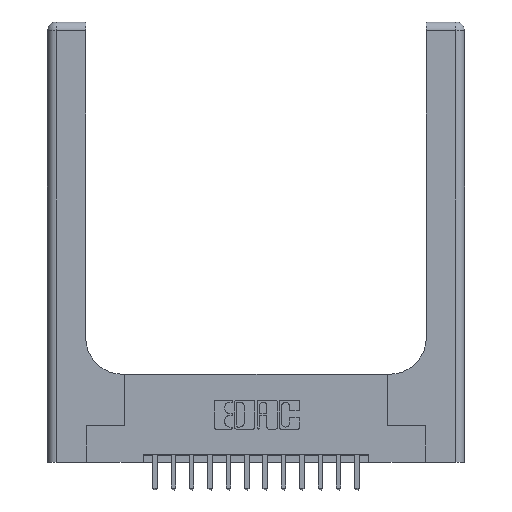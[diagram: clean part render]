
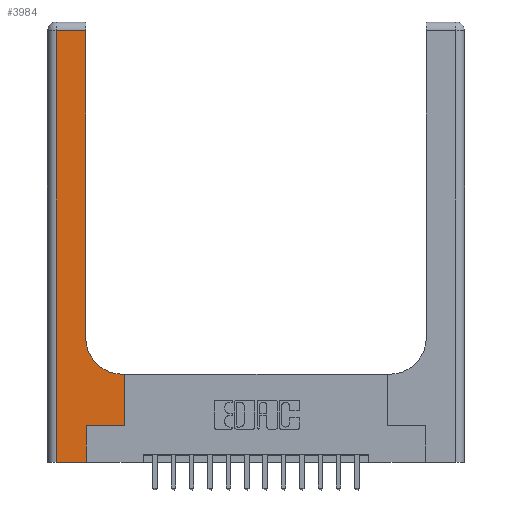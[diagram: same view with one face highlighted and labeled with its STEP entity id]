
A CAD part, top view. The second image highlights one B-rep face of the part: STEP entity #3984.
In plain terms, the highlighted planar face has unit normal (0, 0, 1).
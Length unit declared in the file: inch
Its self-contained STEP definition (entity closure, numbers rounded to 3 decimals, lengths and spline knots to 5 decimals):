
#11 = DIRECTION ( 'NONE',  ( 1., 0., 0. ) ) ;
#186 = LINE ( 'NONE', #16522, #15831 ) ;
#681 = VERTEX_POINT ( 'NONE', #9609 ) ;
#795 = EDGE_LOOP ( 'NONE', ( #807, #1876, #9468, #6690, #6647, #2624, #9070, #843, #6449 ) ) ;
#807 = ORIENTED_EDGE ( 'NONE', *, *, #17196, .T. ) ;
#843 = ORIENTED_EDGE ( 'NONE', *, *, #13848, .T. ) ;
#1026 = DIRECTION ( 'NONE',  ( 0., 1., 0. ) ) ;
#1343 = VERTEX_POINT ( 'NONE', #12396 ) ;
#1766 = DIRECTION ( 'NONE',  ( 0., 1., 0. ) ) ;
#1772 = CARTESIAN_POINT ( 'NONE',  ( 0., 3., 0.37 ) ) ;
#1876 = ORIENTED_EDGE ( 'NONE', *, *, #15842, .T. ) ;
#1943 = LINE ( 'NONE', #8644, #10205 ) ;
#2039 = DIRECTION ( 'NONE',  ( -1., 0., 0. ) ) ;
#2384 = VERTEX_POINT ( 'NONE', #16519 ) ;
#2624 = ORIENTED_EDGE ( 'NONE', *, *, #12705, .T. ) ;
#3038 = CARTESIAN_POINT ( 'NONE',  ( 0., 2.94, 0.37 ) ) ;
#3402 = LINE ( 'NONE', #3038, #15103 ) ;
#3521 = CIRCLE ( 'NONE', #12366, 0.25 ) ;
#3827 = AXIS2_PLACEMENT_3D ( 'NONE', #1772, #5341, #5941 ) ;
#3854 = CARTESIAN_POINT ( 'NONE',  ( 0.26, 3., 0.37 ) ) ;
#3984 = ADVANCED_FACE ( 'NONE', ( #11176 ), #4332, .F. ) ;
#4313 = DIRECTION ( 'NONE',  ( 0., -1., 0. ) ) ;
#4332 = PLANE ( 'NONE',  #3827 ) ;
#4586 = LINE ( 'NONE', #8483, #16909 ) ;
#4690 = CARTESIAN_POINT ( 'NONE',  ( 0.265, 0.25, 0.37 ) ) ;
#5092 = EDGE_CURVE ( 'NONE', #2384, #1343, #3521, .T. ) ;
#5341 = DIRECTION ( 'NONE',  ( 0., 0., -1. ) ) ;
#5524 = VERTEX_POINT ( 'NONE', #4690 ) ;
#5574 = CARTESIAN_POINT ( 'NONE',  ( 0., 0., 0.37 ) ) ;
#5707 = VECTOR ( 'NONE', #7369, 39.37008 ) ;
#5772 = EDGE_CURVE ( 'NONE', #681, #5524, #4586, .T. ) ;
#5941 = DIRECTION ( 'NONE',  ( -1., 0., 0. ) ) ;
#6037 = VERTEX_POINT ( 'NONE', #11807 ) ;
#6064 = EDGE_CURVE ( 'NONE', #12102, #681, #12354, .T. ) ;
#6449 = ORIENTED_EDGE ( 'NONE', *, *, #5092, .T. ) ;
#6647 = ORIENTED_EDGE ( 'NONE', *, *, #5772, .T. ) ;
#6690 = ORIENTED_EDGE ( 'NONE', *, *, #6064, .T. ) ;
#7369 = DIRECTION ( 'NONE',  ( -1., 0., 0. ) ) ;
#7761 = CARTESIAN_POINT ( 'NONE',  ( 0.06, 2.94, 0.37 ) ) ;
#7971 = VERTEX_POINT ( 'NONE', #7761 ) ;
#8050 = VERTEX_POINT ( 'NONE', #14762 ) ;
#8219 = EDGE_CURVE ( 'NONE', #7971, #12102, #186, .T. ) ;
#8483 = CARTESIAN_POINT ( 'NONE',  ( 0.265, 0., 0.37 ) ) ;
#8605 = LINE ( 'NONE', #16819, #5707 ) ;
#8644 = CARTESIAN_POINT ( 'NONE',  ( 0.265, 0.25, 0.37 ) ) ;
#8676 = VECTOR ( 'NONE', #11, 39.37008 ) ;
#9070 = ORIENTED_EDGE ( 'NONE', *, *, #15379, .T. ) ;
#9468 = ORIENTED_EDGE ( 'NONE', *, *, #8219, .T. ) ;
#9609 = CARTESIAN_POINT ( 'NONE',  ( 0.265, 0., 0.37 ) ) ;
#9670 = CARTESIAN_POINT ( 'NONE',  ( 0.26, 2.94, 0.37 ) ) ;
#10205 = VECTOR ( 'NONE', #14080, 39.37008 ) ;
#11176 = FACE_OUTER_BOUND ( 'NONE', #795, .T. ) ;
#11807 = CARTESIAN_POINT ( 'NONE',  ( 0.528, 0.6, 0.37 ) ) ;
#12102 = VERTEX_POINT ( 'NONE', #12962 ) ;
#12287 = VECTOR ( 'NONE', #1026, 39.37008 ) ;
#12354 = LINE ( 'NONE', #5574, #8676 ) ;
#12366 = AXIS2_PLACEMENT_3D ( 'NONE', #17135, #16243, #16161 ) ;
#12396 = CARTESIAN_POINT ( 'NONE',  ( 0.26, 0.85, 0.37 ) ) ;
#12705 = EDGE_CURVE ( 'NONE', #5524, #8050, #1943, .T. ) ;
#12962 = CARTESIAN_POINT ( 'NONE',  ( 0.06, 0., 0.37 ) ) ;
#13123 = LINE ( 'NONE', #3854, #14609 ) ;
#13512 = CARTESIAN_POINT ( 'NONE',  ( 0.528, 0.25, 0.37 ) ) ;
#13848 = EDGE_CURVE ( 'NONE', #6037, #2384, #8605, .T. ) ;
#14080 = DIRECTION ( 'NONE',  ( 1., 0., 0. ) ) ;
#14599 = VERTEX_POINT ( 'NONE', #9670 ) ;
#14609 = VECTOR ( 'NONE', #17115, 39.37008 ) ;
#14762 = CARTESIAN_POINT ( 'NONE',  ( 0.528, 0.25, 0.37 ) ) ;
#15103 = VECTOR ( 'NONE', #2039, 39.37008 ) ;
#15379 = EDGE_CURVE ( 'NONE', #8050, #6037, #17400, .T. ) ;
#15831 = VECTOR ( 'NONE', #4313, 39.37008 ) ;
#15842 = EDGE_CURVE ( 'NONE', #14599, #7971, #3402, .T. ) ;
#16161 = DIRECTION ( 'NONE',  ( 1., 0., 0. ) ) ;
#16243 = DIRECTION ( 'NONE',  ( 0., 0., -1. ) ) ;
#16519 = CARTESIAN_POINT ( 'NONE',  ( 0.51, 0.6, 0.37 ) ) ;
#16522 = CARTESIAN_POINT ( 'NONE',  ( 0.06, 3., 0.37 ) ) ;
#16819 = CARTESIAN_POINT ( 'NONE',  ( 0.26, 0.6, 0.37 ) ) ;
#16909 = VECTOR ( 'NONE', #1766, 39.37008 ) ;
#17115 = DIRECTION ( 'NONE',  ( 0., 1., 0. ) ) ;
#17135 = CARTESIAN_POINT ( 'NONE',  ( 0.51, 0.85, 0.37 ) ) ;
#17196 = EDGE_CURVE ( 'NONE', #1343, #14599, #13123, .T. ) ;
#17400 = LINE ( 'NONE', #13512, #12287 ) ;
